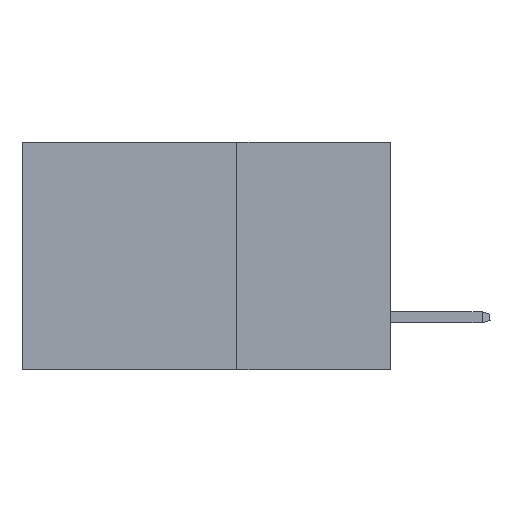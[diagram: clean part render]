
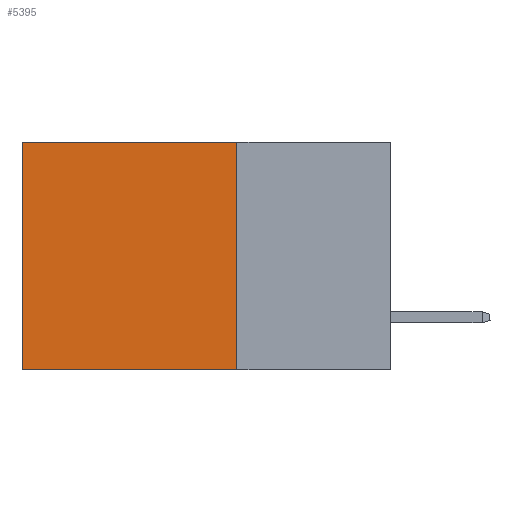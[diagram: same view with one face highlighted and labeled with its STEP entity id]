
A CAD part, left-side view. The second image highlights one B-rep face of the part: STEP entity #5395.
In plain terms, the highlighted planar face has unit normal (-1, 0, 0).
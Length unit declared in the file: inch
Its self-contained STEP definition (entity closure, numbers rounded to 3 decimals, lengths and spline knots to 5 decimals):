
#282 = CARTESIAN_POINT ( 'NONE',  ( 0.2875, 0.25, 0. ) ) ;
#519 = EDGE_CURVE ( 'NONE', #23726, #794, #13211, .T. ) ;
#794 = VERTEX_POINT ( 'NONE', #5965 ) ;
#1440 = AXIS2_PLACEMENT_3D ( 'NONE', #24821, #27038, #13876 ) ;
#2790 = CARTESIAN_POINT ( 'NONE',  ( 0.2875, 0.25, 0. ) ) ;
#5395 = ADVANCED_FACE ( 'NONE', ( #22395 ), #20325, .F. ) ;
#5965 = CARTESIAN_POINT ( 'NONE',  ( 0.2875, 0.6, 0. ) ) ;
#9558 = LINE ( 'NONE', #12609, #16478 ) ;
#10097 = DIRECTION ( 'NONE',  ( 0., 1., 0. ) ) ;
#10356 = ORIENTED_EDGE ( 'NONE', *, *, #11309, .T. ) ;
#11137 = VERTEX_POINT ( 'NONE', #12026 ) ;
#11309 = EDGE_CURVE ( 'NONE', #794, #16262, #24695, .T. ) ;
#11342 = EDGE_CURVE ( 'NONE', #23726, #11137, #18524, .T. ) ;
#11489 = DIRECTION ( 'NONE',  ( 0., 1., 0. ) ) ;
#12026 = CARTESIAN_POINT ( 'NONE',  ( 0.2875, 0.25, -0.37 ) ) ;
#12596 = ORIENTED_EDGE ( 'NONE', *, *, #19106, .F. ) ;
#12609 = CARTESIAN_POINT ( 'NONE',  ( 0.2875, 0.25, -0.37 ) ) ;
#12660 = CARTESIAN_POINT ( 'NONE',  ( 0.2875, 0.6, 0. ) ) ;
#13211 = LINE ( 'NONE', #2790, #24193 ) ;
#13876 = DIRECTION ( 'NONE',  ( 0., 0., -1. ) ) ;
#16262 = VERTEX_POINT ( 'NONE', #24303 ) ;
#16478 = VECTOR ( 'NONE', #10097, 39.37008 ) ;
#17333 = DIRECTION ( 'NONE',  ( 0., 0., -1. ) ) ;
#18102 = DIRECTION ( 'NONE',  ( 0., 0., -1. ) ) ;
#18524 = LINE ( 'NONE', #28071, #26111 ) ;
#18686 = ORIENTED_EDGE ( 'NONE', *, *, #11342, .F. ) ;
#19061 = ORIENTED_EDGE ( 'NONE', *, *, #519, .T. ) ;
#19106 = EDGE_CURVE ( 'NONE', #11137, #16262, #9558, .T. ) ;
#20254 = VECTOR ( 'NONE', #17333, 39.37008 ) ;
#20325 = PLANE ( 'NONE',  #1440 ) ;
#22395 = FACE_OUTER_BOUND ( 'NONE', #24962, .T. ) ;
#23726 = VERTEX_POINT ( 'NONE', #282 ) ;
#24193 = VECTOR ( 'NONE', #11489, 39.37008 ) ;
#24303 = CARTESIAN_POINT ( 'NONE',  ( 0.2875, 0.6, -0.37 ) ) ;
#24695 = LINE ( 'NONE', #12660, #20254 ) ;
#24821 = CARTESIAN_POINT ( 'NONE',  ( 0.2875, 0.25, 0. ) ) ;
#24962 = EDGE_LOOP ( 'NONE', ( #10356, #12596, #18686, #19061 ) ) ;
#26111 = VECTOR ( 'NONE', #18102, 39.37008 ) ;
#27038 = DIRECTION ( 'NONE',  ( 1., 0., 0. ) ) ;
#28071 = CARTESIAN_POINT ( 'NONE',  ( 0.2875, 0.25, 0. ) ) ;
